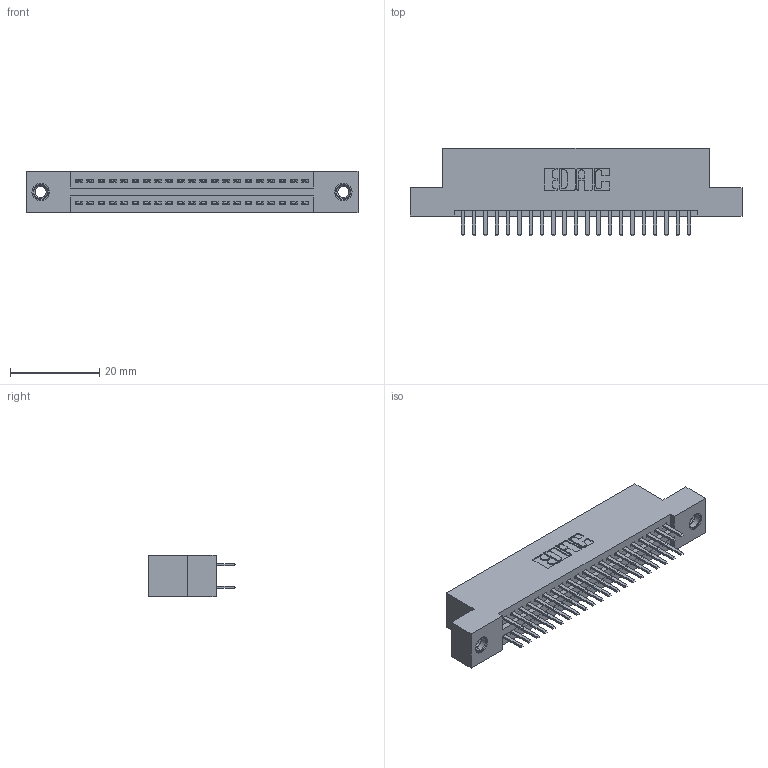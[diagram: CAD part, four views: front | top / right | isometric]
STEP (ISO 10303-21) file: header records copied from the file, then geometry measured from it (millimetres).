
FILE_DESCRIPTION (( 'STEP AP203' ), '1' );
FILE_NAME ('345-042-520-207.STEP', '2018-09-05T10:37:41', ( '' ), ( '' ), 'SwSTEP 2.0', 'SolidWorks 2016', '' );
FILE_SCHEMA (( 'CONFIG_CONTROL_DESIGN' ));
Length unit declared in the file: inch
Products named in the file (4): 345-042-520-207; 345 Part_Flush Mounting Lugs - 0.156 Dia-TI; 345-292-001_345-293-120; 345-250-001_345-250-005-103
Assembly tree (45 placements, depth 2):
  345-042-520-207
    345 Part_Flush Mounting Lugs - 0.156 Dia-TI
    345-292-001_345-293-120  x42
    345-250-001_345-250-005-103  x2
Bounding box: 74.55 x 19.68 x 9.4 mm (x, y, z)
Volume: 7014.9 mm3; surface area: 9951 mm2
Topology: 45 solids, 45 shells, 2454 faces, 7071 edges, 4594 vertices
Faces by surface type: plane 1582, cylinder 856, cone 12, torus 4
Entity records: 20604 total; most frequent: CARTESIAN_POINT 3467, ORIENTED_EDGE 3382, DIRECTION 3097, EDGE_CURVE 1691, VECTOR 1451, LINE 1451, VERTEX_POINT 1120, AXIS2_PLACEMENT_3D 823
